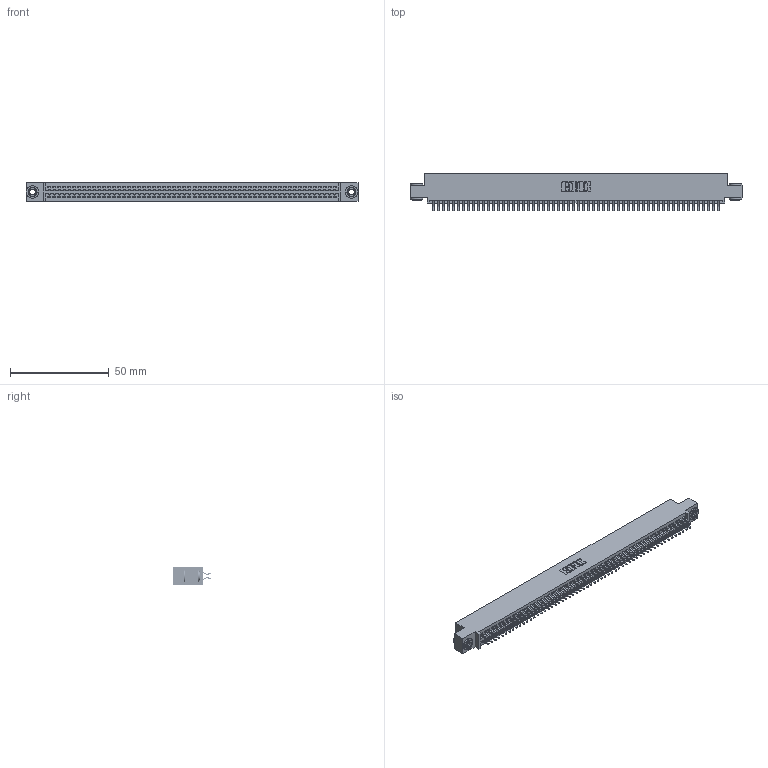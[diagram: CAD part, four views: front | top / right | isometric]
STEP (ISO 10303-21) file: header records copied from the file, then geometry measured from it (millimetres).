
FILE_DESCRIPTION (( 'STEP AP203' ), '1' );
FILE_NAME ('345-116-556-503.STEP', '2019-11-05T16:43:39', ( '' ), ( '' ), 'SwSTEP 2.0', 'SolidWorks 2016', '' );
FILE_SCHEMA (( 'CONFIG_CONTROL_DESIGN' ));
Length unit declared in the file: inch
Products named in the file (4): 345-292-001_556 Tail; 345-250-002_345-250-002-102; 345 Part_0.110 Offset - 0.156 Dia-TH; 345-116-556-503
Assembly tree (119 placements, depth 2):
  345-116-556-503
    345 Part_0.110 Offset - 0.156 Dia-TH
    345-292-001_556 Tail  x116
    345-250-002_345-250-002-102  x2
Bounding box: 168.53 x 19.24 x 9.4 mm (x, y, z)
Volume: 16461 mm3; surface area: 24838.2 mm2
Topology: 119 solids, 119 shells, 6664 faces, 19801 edges, 13042 vertices
Faces by surface type: plane 4386, cylinder 2270, cone 8
Entity records: 44356 total; most frequent: CARTESIAN_POINT 7411, ORIENTED_EDGE 7326, DIRECTION 6533, EDGE_CURVE 3663, VECTOR 3267, LINE 3267, VERTEX_POINT 2438, AXIS2_PLACEMENT_3D 1633
